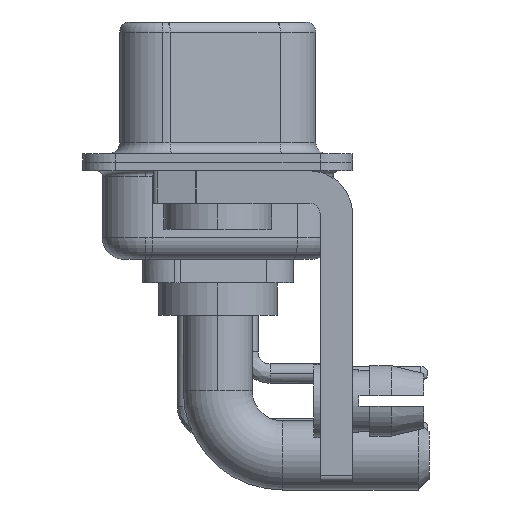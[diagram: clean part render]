
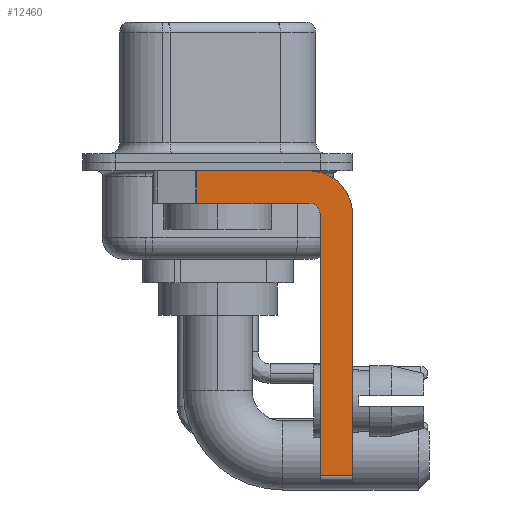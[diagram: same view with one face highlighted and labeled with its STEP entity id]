
A CAD part, left-side view. The second image highlights one B-rep face of the part: STEP entity #12460.
In plain terms, the highlighted planar face has unit normal (-1, 0, 0).
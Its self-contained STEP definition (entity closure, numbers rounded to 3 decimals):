
#150 = DIRECTION ( 'NONE',  ( 0., -1., 0. ) ) ;
#471 = ORIENTED_EDGE ( 'NONE', *, *, #10552, .F. ) ;
#776 = CARTESIAN_POINT ( 'NONE',  ( -2.9, -6.25, -2.4 ) ) ;
#1389 = CARTESIAN_POINT ( 'NONE',  ( -2.9, 0.978, -0.4 ) ) ;
#1501 = LINE ( 'NONE', #3684, #20051 ) ;
#1835 = EDGE_CURVE ( 'NONE', #24732, #4785, #25952, .T. ) ;
#2143 = EDGE_LOOP ( 'NONE', ( #471, #26078, #8103, #2702, #22588, #16590, #9247, #22843 ) ) ;
#2389 = AXIS2_PLACEMENT_3D ( 'NONE', #11635, #9179, #11237 ) ;
#2702 = ORIENTED_EDGE ( 'NONE', *, *, #21295, .F. ) ;
#2867 = CARTESIAN_POINT ( 'NONE',  ( -2.9, 0.978, -1.9 ) ) ;
#3684 = CARTESIAN_POINT ( 'NONE',  ( -2.9, 3., -0.4 ) ) ;
#4220 = VERTEX_POINT ( 'NONE', #2867 ) ;
#4785 = VERTEX_POINT ( 'NONE', #11565 ) ;
#5296 = VECTOR ( 'NONE', #150, 1000. ) ;
#5379 = DIRECTION ( 'NONE',  ( 0., 0., -1. ) ) ;
#5431 = DIRECTION ( 'NONE',  ( 0., 1., 0. ) ) ;
#5455 = CARTESIAN_POINT ( 'NONE',  ( -2.9, -4.75, -14.8 ) ) ;
#5521 = CARTESIAN_POINT ( 'NONE',  ( -2.9, -6.25, -14.55 ) ) ;
#6426 = DIRECTION ( 'NONE',  ( 0., 0., -1. ) ) ;
#6503 = VECTOR ( 'NONE', #26278, 1000. ) ;
#7048 = DIRECTION ( 'NONE',  ( 0., 0., -1. ) ) ;
#7401 = VERTEX_POINT ( 'NONE', #12512 ) ;
#7573 = AXIS2_PLACEMENT_3D ( 'NONE', #17465, #11541, #5379 ) ;
#7607 = CARTESIAN_POINT ( 'NONE',  ( -2.9, -4.75, -2.4 ) ) ;
#8103 = ORIENTED_EDGE ( 'NONE', *, *, #24546, .F. ) ;
#9179 = DIRECTION ( 'NONE',  ( -1., 0., 0. ) ) ;
#9247 = ORIENTED_EDGE ( 'NONE', *, *, #17695, .F. ) ;
#9388 = LINE ( 'NONE', #23776, #20908 ) ;
#10434 = EDGE_CURVE ( 'NONE', #7401, #13213, #18204, .T. ) ;
#10521 = CARTESIAN_POINT ( 'NONE',  ( -2.9, -4.25, -14.55 ) ) ;
#10552 = EDGE_CURVE ( 'NONE', #13691, #24732, #1501, .T. ) ;
#11237 = DIRECTION ( 'NONE',  ( 0., 0., 1. ) ) ;
#11541 = DIRECTION ( 'NONE',  ( 1., 0., 0. ) ) ;
#11565 = CARTESIAN_POINT ( 'NONE',  ( -2.9, -6.25, -2.4 ) ) ;
#11635 = CARTESIAN_POINT ( 'NONE',  ( -2.9, -4.25, -2.4 ) ) ;
#12023 = DIRECTION ( 'NONE',  ( 0., -1., 0. ) ) ;
#12178 = LINE ( 'NONE', #10521, #5296 ) ;
#12460 = ADVANCED_FACE ( 'NONE', ( #22309 ), #17949, .F. ) ;
#12471 = VERTEX_POINT ( 'NONE', #20667 ) ;
#12512 = CARTESIAN_POINT ( 'NONE',  ( -2.9, -4.75, -14.55 ) ) ;
#12544 = EDGE_CURVE ( 'NONE', #7401, #17926, #12178, .T. ) ;
#13213 = VERTEX_POINT ( 'NONE', #7607 ) ;
#13227 = EDGE_CURVE ( 'NONE', #13691, #4220, #9388, .T. ) ;
#13691 = VERTEX_POINT ( 'NONE', #1389 ) ;
#15370 = VECTOR ( 'NONE', #7048, 1000. ) ;
#16590 = ORIENTED_EDGE ( 'NONE', *, *, #12544, .T. ) ;
#17465 = CARTESIAN_POINT ( 'NONE',  ( -2.9, -4.25, -2.4 ) ) ;
#17695 = EDGE_CURVE ( 'NONE', #4785, #17926, #19515, .T. ) ;
#17926 = VERTEX_POINT ( 'NONE', #5521 ) ;
#17949 = PLANE ( 'NONE',  #18846 ) ;
#18142 = CIRCLE ( 'NONE', #2389, 0.5 ) ;
#18204 = LINE ( 'NONE', #5455, #6503 ) ;
#18666 = VECTOR ( 'NONE', #5431, 1000. ) ;
#18846 = AXIS2_PLACEMENT_3D ( 'NONE', #26300, #23138, #6426 ) ;
#19515 = LINE ( 'NONE', #776, #15370 ) ;
#20051 = VECTOR ( 'NONE', #12023, 1000. ) ;
#20667 = CARTESIAN_POINT ( 'NONE',  ( -2.9, -4.25, -1.9 ) ) ;
#20908 = VECTOR ( 'NONE', #24312, 1000. ) ;
#21295 = EDGE_CURVE ( 'NONE', #13213, #12471, #18142, .T. ) ;
#22309 = FACE_OUTER_BOUND ( 'NONE', #2143, .T. ) ;
#22588 = ORIENTED_EDGE ( 'NONE', *, *, #10434, .F. ) ;
#22843 = ORIENTED_EDGE ( 'NONE', *, *, #1835, .F. ) ;
#23138 = DIRECTION ( 'NONE',  ( 1., 0., 0. ) ) ;
#23776 = CARTESIAN_POINT ( 'NONE',  ( -2.9, 0.978, -1.9 ) ) ;
#24192 = LINE ( 'NONE', #26392, #18666 ) ;
#24312 = DIRECTION ( 'NONE',  ( 0., 0., -1. ) ) ;
#24546 = EDGE_CURVE ( 'NONE', #12471, #4220, #24192, .T. ) ;
#24732 = VERTEX_POINT ( 'NONE', #26657 ) ;
#25952 = CIRCLE ( 'NONE', #7573, 2. ) ;
#26078 = ORIENTED_EDGE ( 'NONE', *, *, #13227, .T. ) ;
#26278 = DIRECTION ( 'NONE',  ( 0., 0., 1. ) ) ;
#26300 = CARTESIAN_POINT ( 'NONE',  ( -2.9, -4.25, -2.4 ) ) ;
#26392 = CARTESIAN_POINT ( 'NONE',  ( -2.9, -4.25, -1.9 ) ) ;
#26657 = CARTESIAN_POINT ( 'NONE',  ( -2.9, -4.25, -0.4 ) ) ;
